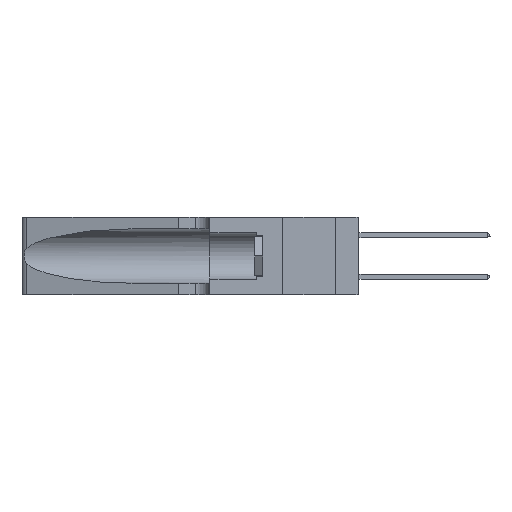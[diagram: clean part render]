
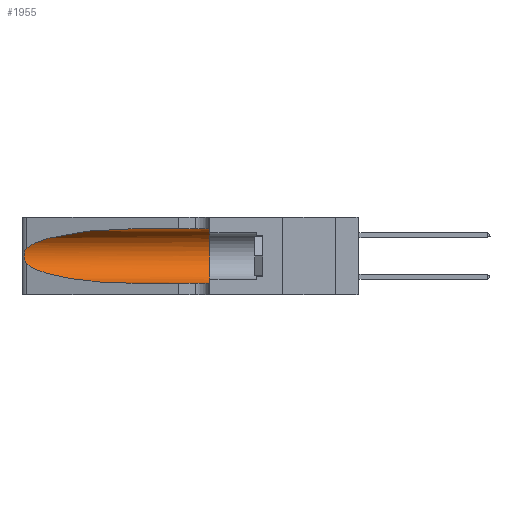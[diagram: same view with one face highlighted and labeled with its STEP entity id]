
A CAD part, left-side view. The second image highlights one B-rep face of the part: STEP entity #1955.
In plain terms, the highlighted cylindrical face has radius 3.308 mm (diameter 6.617 mm), a partial arc.
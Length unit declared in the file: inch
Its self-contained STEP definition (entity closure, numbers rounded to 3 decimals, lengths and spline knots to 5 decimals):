
#940 = DIRECTION ( 'NONE',  ( 0., -1., 0. ) ) ;
#1743 = CARTESIAN_POINT ( 'NONE',  ( 0.25856, 1.23593, 0.16098 ) ) ;
#1955 = ADVANCED_FACE ( 'NONE', ( #3348 ), #14573, .F. ) ;
#3348 = FACE_OUTER_BOUND ( 'NONE', #5331, .T. ) ;
#4278 = CARTESIAN_POINT ( 'NONE',  ( 0.1305, 1.61858, 0.05475 ) ) ;
#4894 = CARTESIAN_POINT ( 'NONE',  ( 0.26075, 1.23896, 0.19203 ) ) ;
#4925 = ORIENTED_EDGE ( 'NONE', *, *, #21523, .T. ) ;
#5187 = CARTESIAN_POINT ( 'NONE',  ( 0.25854, 1.2359, 0.20912 ) ) ;
#5331 = EDGE_LOOP ( 'NONE', ( #11915, #8402, #26443, #4925, #41486, #16866 ) ) ;
#5939 = VECTOR ( 'NONE', #37065, 39.37008 ) ;
#6642 = LINE ( 'NONE', #4278, #41984 ) ;
#6684 = DIRECTION ( 'NONE',  ( 0., -1., 0. ) ) ;
#7713 = VERTEX_POINT ( 'NONE', #35675 ) ;
#8402 = ORIENTED_EDGE ( 'NONE', *, *, #36276, .T. ) ;
#9284 = DIRECTION ( 'NONE',  ( 0., 1., 0. ) ) ;
#11201 = CARTESIAN_POINT ( 'NONE',  ( 0.18966, 0.96281, 0.31525 ) ) ;
#11464 = CARTESIAN_POINT ( 'NONE',  ( 0.26075, 1.23896, 0.178 ) ) ;
#11915 = ORIENTED_EDGE ( 'NONE', *, *, #18295, .T. ) ;
#12094 = CARTESIAN_POINT ( 'NONE',  ( 0.25555, 1.22993, 0.14849 ) ) ;
#12380 = AXIS2_PLACEMENT_3D ( 'NONE', #33091, #9284, #22727 ) ;
#14330 = CARTESIAN_POINT ( 'NONE',  ( 0.18966, 0.96281, 0.05475 ) ) ;
#14573 = CYLINDRICAL_SURFACE ( 'NONE', #35591, 0.13025 ) ;
#14824 = CARTESIAN_POINT ( 'NONE',  ( 0.25487, 1.22718, 0.22369 ) ) ;
#14928 = CARTESIAN_POINT ( 'NONE',  ( 0.26018, 1.23835, 0.19895 ) ) ;
#15091 = CARTESIAN_POINT ( 'NONE',  ( 0.25487, 1.22718, 0.14631 ) ) ;
#16808 = CARTESIAN_POINT ( 'NONE',  ( 0.1305, 0.72297, 0.05475 ) ) ;
#16866 = ORIENTED_EDGE ( 'NONE', *, *, #38405, .F. ) ;
#17013 = CARTESIAN_POINT ( 'NONE',  ( 0.1305, 1.61858, 0.185 ) ) ;
#18295 = EDGE_CURVE ( 'NONE', #19558, #43366, #30865, .T. ) ;
#18881 = VERTEX_POINT ( 'NONE', #23342 ) ;
#19558 = VERTEX_POINT ( 'NONE', #23141 ) ;
#20579 = DIRECTION ( 'NONE',  ( 0., 0., -1. ) ) ;
#21019 = CARTESIAN_POINT ( 'NONE',  ( 0.25487, 1.22718, 0.14631 ) ) ;
#21523 = EDGE_CURVE ( 'NONE', #30340, #7713, #6642, .T. ) ;
#22060 = CARTESIAN_POINT ( 'NONE',  ( 0.25555, 1.22994, 0.2215 ) ) ;
#22223 = CARTESIAN_POINT ( 'NONE',  ( 0.25639, 1.23184, 0.21858 ) ) ;
#22727 = DIRECTION ( 'NONE',  ( 0., 0., 1. ) ) ;
#23141 = CARTESIAN_POINT ( 'NONE',  ( 0.1305, 0.72297, 0.31525 ) ) ;
#23342 = CARTESIAN_POINT ( 'NONE',  ( 0.25487, 1.22718, 0.14631 ) ) ;
#23561 = CARTESIAN_POINT ( 'NONE',  ( 0.1305, 1.61858, 0.31525 ) ) ;
#25393 = CARTESIAN_POINT ( 'NONE',  ( 0.25639, 1.23186, 0.15144 ) ) ;
#25704 = CARTESIAN_POINT ( 'NONE',  ( 0.25789, 1.23486, 0.15765 ) ) ;
#26443 = ORIENTED_EDGE ( 'NONE', *, *, #39993, .T. ) ;
#26779 = B_SPLINE_CURVE_WITH_KNOTS ( 'NONE', 3,
 ( #31971, #22060, #22223, #38848, #5187, #14928, #4894, #11464, #35561, #1743, #25704, #25393, #12094, #15091 ),
 .UNSPECIFIED., .F., .F.,
 ( 4, 2, 2, 2, 2, 2, 4 ),
 ( 0., 0.00027, 0.00053, 0.00107, 0.0016, 0.00187, 0.00214 ),
 .UNSPECIFIED. ) ;
#27836 = LINE ( 'NONE', #23561, #5939 ) ;
#29803 = CIRCLE ( 'NONE', #12380, 0.13025 ) ;
#30090 =( BOUNDED_CURVE ( )  B_SPLINE_CURVE ( 3, ( #21019, #34811, #14330, #41704 ),
 .UNSPECIFIED., .F., .T. ) 
 B_SPLINE_CURVE_WITH_KNOTS ( ( 4, 4 ),
 ( 3.44316, 4.71239 ),
 .UNSPECIFIED. ) 
 CURVE ( )  GEOMETRIC_REPRESENTATION_ITEM ( )  RATIONAL_B_SPLINE_CURVE ( ( 1., 0.87, 0.87, 1. ) ) 
 REPRESENTATION_ITEM ( '' )  );
#30340 = VERTEX_POINT ( 'NONE', #16808 ) ;
#30865 =( BOUNDED_CURVE ( )  B_SPLINE_CURVE ( 3, ( #35447, #11201, #31863, #14824 ),
 .UNSPECIFIED., .F., .F. ) 
 B_SPLINE_CURVE_WITH_KNOTS ( ( 4, 4 ),
 ( 1.5708, 2.84003 ),
 .UNSPECIFIED. ) 
 CURVE ( )  GEOMETRIC_REPRESENTATION_ITEM ( )  RATIONAL_B_SPLINE_CURVE ( ( 1., 0.87, 0.87, 1. ) ) 
 REPRESENTATION_ITEM ( '' )  );
#31863 = CARTESIAN_POINT ( 'NONE',  ( 0.2373, 1.15595, 0.28018 ) ) ;
#31971 = CARTESIAN_POINT ( 'NONE',  ( 0.25487, 1.22718, 0.22369 ) ) ;
#33091 = CARTESIAN_POINT ( 'NONE',  ( 0.1305, 0.35, 0.185 ) ) ;
#34811 = CARTESIAN_POINT ( 'NONE',  ( 0.2373, 1.15595, 0.08982 ) ) ;
#34889 = CARTESIAN_POINT ( 'NONE',  ( 0.25487, 1.22718, 0.22369 ) ) ;
#35447 = CARTESIAN_POINT ( 'NONE',  ( 0.1305, 0.72297, 0.31525 ) ) ;
#35561 = CARTESIAN_POINT ( 'NONE',  ( 0.26017, 1.23833, 0.17102 ) ) ;
#35591 = AXIS2_PLACEMENT_3D ( 'NONE', #17013, #6684, #20579 ) ;
#35675 = CARTESIAN_POINT ( 'NONE',  ( 0.1305, 0.35, 0.05475 ) ) ;
#36276 = EDGE_CURVE ( 'NONE', #43366, #18881, #26779, .T. ) ;
#36468 = CARTESIAN_POINT ( 'NONE',  ( 0.1305, 0.35, 0.31525 ) ) ;
#37065 = DIRECTION ( 'NONE',  ( 0., -1., 0. ) ) ;
#38227 = VERTEX_POINT ( 'NONE', #36468 ) ;
#38405 = EDGE_CURVE ( 'NONE', #19558, #38227, #27836, .T. ) ;
#38848 = CARTESIAN_POINT ( 'NONE',  ( 0.25787, 1.23484, 0.2124 ) ) ;
#39993 = EDGE_CURVE ( 'NONE', #18881, #30340, #30090, .T. ) ;
#41486 = ORIENTED_EDGE ( 'NONE', *, *, #41573, .F. ) ;
#41573 = EDGE_CURVE ( 'NONE', #38227, #7713, #29803, .T. ) ;
#41704 = CARTESIAN_POINT ( 'NONE',  ( 0.1305, 0.72297, 0.05475 ) ) ;
#41984 = VECTOR ( 'NONE', #940, 39.37008 ) ;
#43366 = VERTEX_POINT ( 'NONE', #34889 ) ;
